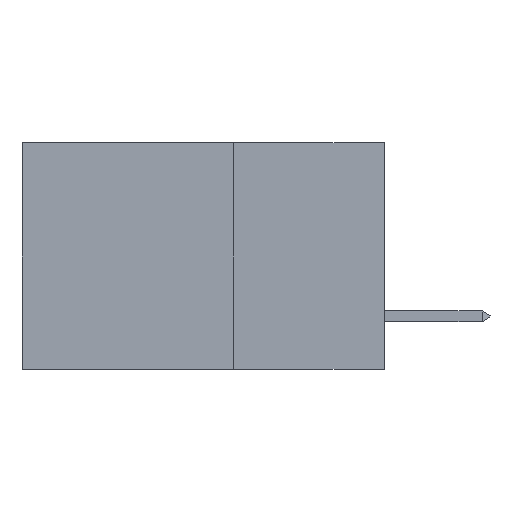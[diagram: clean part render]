
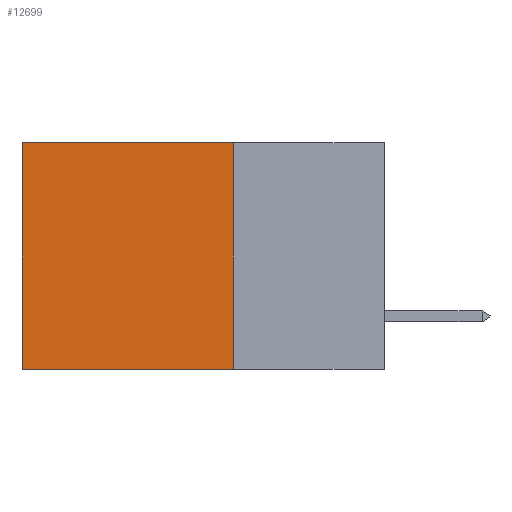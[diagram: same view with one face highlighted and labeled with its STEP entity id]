
A CAD part, left-side view. The second image highlights one B-rep face of the part: STEP entity #12699.
In plain terms, the highlighted planar face has unit normal (-1, 0, 0).
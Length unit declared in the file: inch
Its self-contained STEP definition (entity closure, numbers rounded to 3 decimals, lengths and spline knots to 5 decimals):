
#460 = DIRECTION ( 'NONE',  ( 0., 1., 0. ) ) ;
#1176 = VECTOR ( 'NONE', #14490, 39.37008 ) ;
#1179 = CARTESIAN_POINT ( 'NONE',  ( 0.2875, 0.25, 0. ) ) ;
#1201 = EDGE_CURVE ( 'NONE', #5448, #2355, #10544, .T. ) ;
#1265 = DIRECTION ( 'NONE',  ( 0., 0., -1. ) ) ;
#1835 = EDGE_LOOP ( 'NONE', ( #14859, #3529, #13547, #2210 ) ) ;
#2210 = ORIENTED_EDGE ( 'NONE', *, *, #11801, .T. ) ;
#2355 = VERTEX_POINT ( 'NONE', #14834 ) ;
#2936 = FACE_OUTER_BOUND ( 'NONE', #1835, .T. ) ;
#2952 = VECTOR ( 'NONE', #7620, 39.37008 ) ;
#3029 = EDGE_CURVE ( 'NONE', #12000, #10845, #12905, .T. ) ;
#3529 = ORIENTED_EDGE ( 'NONE', *, *, #12382, .F. ) ;
#3871 = CARTESIAN_POINT ( 'NONE',  ( 0.2875, 0.25, -0.375 ) ) ;
#4292 = VECTOR ( 'NONE', #14563, 39.37008 ) ;
#5175 = CARTESIAN_POINT ( 'NONE',  ( 0.2875, 0.25, 0. ) ) ;
#5448 = VERTEX_POINT ( 'NONE', #14396 ) ;
#6340 = CARTESIAN_POINT ( 'NONE',  ( 0.2875, 0.6, -0.375 ) ) ;
#7205 = AXIS2_PLACEMENT_3D ( 'NONE', #11652, #8143, #1265 ) ;
#7360 = CARTESIAN_POINT ( 'NONE',  ( 0.2875, 0.25, -0.375 ) ) ;
#7620 = DIRECTION ( 'NONE',  ( 0., 1., 0. ) ) ;
#8130 = VECTOR ( 'NONE', #460, 39.37008 ) ;
#8143 = DIRECTION ( 'NONE',  ( 1., 0., 0. ) ) ;
#8646 = LINE ( 'NONE', #3871, #2952 ) ;
#10458 = CARTESIAN_POINT ( 'NONE',  ( 0.2875, 0.25, -0.375 ) ) ;
#10544 = LINE ( 'NONE', #6340, #4292 ) ;
#10845 = VERTEX_POINT ( 'NONE', #10458 ) ;
#11652 = CARTESIAN_POINT ( 'NONE',  ( 0.2875, 0.25, -0.375 ) ) ;
#11796 = PLANE ( 'NONE',  #7205 ) ;
#11801 = EDGE_CURVE ( 'NONE', #12000, #5448, #12490, .T. ) ;
#12000 = VERTEX_POINT ( 'NONE', #1179 ) ;
#12382 = EDGE_CURVE ( 'NONE', #10845, #2355, #8646, .T. ) ;
#12490 = LINE ( 'NONE', #5175, #8130 ) ;
#12699 = ADVANCED_FACE ( 'NONE', ( #2936 ), #11796, .F. ) ;
#12905 = LINE ( 'NONE', #7360, #1176 ) ;
#13547 = ORIENTED_EDGE ( 'NONE', *, *, #3029, .F. ) ;
#14396 = CARTESIAN_POINT ( 'NONE',  ( 0.2875, 0.6, 0. ) ) ;
#14490 = DIRECTION ( 'NONE',  ( 0., 0., -1. ) ) ;
#14563 = DIRECTION ( 'NONE',  ( 0., 0., -1. ) ) ;
#14834 = CARTESIAN_POINT ( 'NONE',  ( 0.2875, 0.6, -0.375 ) ) ;
#14859 = ORIENTED_EDGE ( 'NONE', *, *, #1201, .T. ) ;
